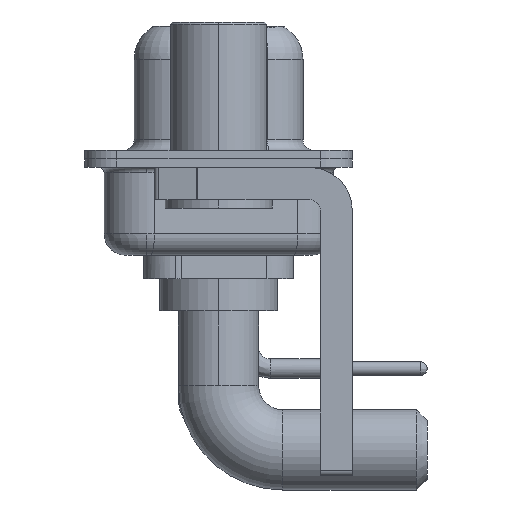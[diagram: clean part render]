
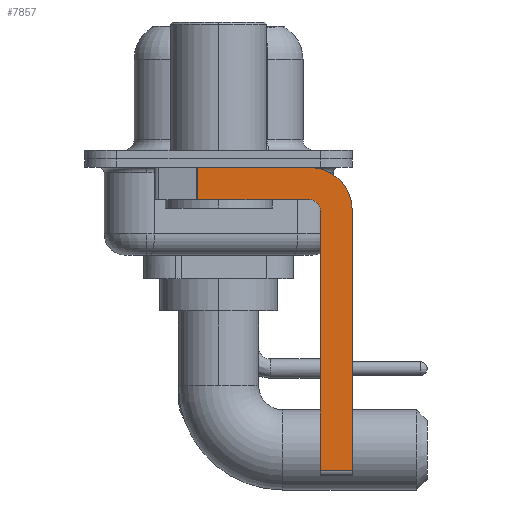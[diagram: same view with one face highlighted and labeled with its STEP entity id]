
A CAD part, left-side view. The second image highlights one B-rep face of the part: STEP entity #7857.
In plain terms, the highlighted planar face has unit normal (-1, 0, 0).
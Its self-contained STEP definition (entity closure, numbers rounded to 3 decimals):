
#25 = CARTESIAN_POINT ( 'NONE',  ( -2.9, -4.25, -0.4 ) ) ;
#339 = CARTESIAN_POINT ( 'NONE',  ( -2.9, -6.25, -2.4 ) ) ;
#407 = VERTEX_POINT ( 'NONE', #7851 ) ;
#475 = VECTOR ( 'NONE', #18164, 1000. ) ;
#522 = CIRCLE ( 'NONE', #15997, 2. ) ;
#2078 = VECTOR ( 'NONE', #6536, 1000. ) ;
#2760 = DIRECTION ( 'NONE',  ( 0., 0., 1. ) ) ;
#2777 = DIRECTION ( 'NONE',  ( 1., 0., 0. ) ) ;
#3137 = ORIENTED_EDGE ( 'NONE', *, *, #11200, .F. ) ;
#3430 = DIRECTION ( 'NONE',  ( 1., 0., 0. ) ) ;
#3454 = DIRECTION ( 'NONE',  ( 0., 0., 1. ) ) ;
#3721 = VERTEX_POINT ( 'NONE', #17785 ) ;
#4011 = EDGE_CURVE ( 'NONE', #407, #14669, #10313, .T. ) ;
#4802 = EDGE_CURVE ( 'NONE', #6082, #14540, #522, .T. ) ;
#5266 = VECTOR ( 'NONE', #23229, 1000. ) ;
#5614 = VECTOR ( 'NONE', #20807, 1000. ) ;
#6082 = VERTEX_POINT ( 'NONE', #25 ) ;
#6085 = DIRECTION ( 'NONE',  ( -1., 0., 0. ) ) ;
#6464 = EDGE_CURVE ( 'NONE', #15797, #6748, #22939, .T. ) ;
#6536 = DIRECTION ( 'NONE',  ( 0., -1., 0. ) ) ;
#6683 = CARTESIAN_POINT ( 'NONE',  ( -2.9, -4.25, -2.4 ) ) ;
#6748 = VERTEX_POINT ( 'NONE', #16519 ) ;
#6986 = DIRECTION ( 'NONE',  ( 0., 1., 0. ) ) ;
#6990 = DIRECTION ( 'NONE',  ( 0., 0., -1. ) ) ;
#7174 = CARTESIAN_POINT ( 'NONE',  ( -2.9, -6.25, -2.4 ) ) ;
#7233 = CARTESIAN_POINT ( 'NONE',  ( -2.9, -4.75, -14.8 ) ) ;
#7406 = EDGE_CURVE ( 'NONE', #15797, #6082, #21449, .T. ) ;
#7851 = CARTESIAN_POINT ( 'NONE',  ( -2.9, -4.75, -2.4 ) ) ;
#7857 = ADVANCED_FACE ( 'NONE', ( #15652 ), #22893, .F. ) ;
#8286 = AXIS2_PLACEMENT_3D ( 'NONE', #6683, #2777, #18986 ) ;
#9037 = ORIENTED_EDGE ( 'NONE', *, *, #7406, .F. ) ;
#10070 = CARTESIAN_POINT ( 'NONE',  ( -2.9, 0.978, -0.4 ) ) ;
#10183 = EDGE_CURVE ( 'NONE', #19823, #407, #23227, .T. ) ;
#10247 = ORIENTED_EDGE ( 'NONE', *, *, #10538, .F. ) ;
#10313 = CIRCLE ( 'NONE', #14113, 0.5 ) ;
#10538 = EDGE_CURVE ( 'NONE', #14669, #6748, #12653, .T. ) ;
#11200 = EDGE_CURVE ( 'NONE', #14540, #3721, #19838, .T. ) ;
#11345 = VECTOR ( 'NONE', #6986, 1000. ) ;
#12142 = CARTESIAN_POINT ( 'NONE',  ( -2.9, 0.978, -1.9 ) ) ;
#12621 = ORIENTED_EDGE ( 'NONE', *, *, #10183, .F. ) ;
#12632 = CARTESIAN_POINT ( 'NONE',  ( -2.9, -4.75, -14.55 ) ) ;
#12653 = LINE ( 'NONE', #17727, #11345 ) ;
#12671 = ORIENTED_EDGE ( 'NONE', *, *, #15857, .T. ) ;
#14113 = AXIS2_PLACEMENT_3D ( 'NONE', #22279, #6085, #2760 ) ;
#14417 = CARTESIAN_POINT ( 'NONE',  ( -2.9, -4.25, -2.4 ) ) ;
#14540 = VERTEX_POINT ( 'NONE', #339 ) ;
#14669 = VERTEX_POINT ( 'NONE', #19959 ) ;
#14674 = CARTESIAN_POINT ( 'NONE',  ( -2.9, 3., -0.4 ) ) ;
#15652 = FACE_OUTER_BOUND ( 'NONE', #16836, .T. ) ;
#15797 = VERTEX_POINT ( 'NONE', #10070 ) ;
#15857 = EDGE_CURVE ( 'NONE', #19823, #3721, #19074, .T. ) ;
#15997 = AXIS2_PLACEMENT_3D ( 'NONE', #14417, #3430, #6990 ) ;
#16519 = CARTESIAN_POINT ( 'NONE',  ( -2.9, 0.978, -1.9 ) ) ;
#16836 = EDGE_LOOP ( 'NONE', ( #9037, #17601, #10247, #20373, #12621, #12671, #3137, #21345 ) ) ;
#17601 = ORIENTED_EDGE ( 'NONE', *, *, #6464, .T. ) ;
#17727 = CARTESIAN_POINT ( 'NONE',  ( -2.9, -4.25, -1.9 ) ) ;
#17785 = CARTESIAN_POINT ( 'NONE',  ( -2.9, -6.25, -14.55 ) ) ;
#18164 = DIRECTION ( 'NONE',  ( 0., 0., -1. ) ) ;
#18986 = DIRECTION ( 'NONE',  ( 0., 0., -1. ) ) ;
#19074 = LINE ( 'NONE', #22744, #2078 ) ;
#19823 = VERTEX_POINT ( 'NONE', #12632 ) ;
#19838 = LINE ( 'NONE', #7174, #475 ) ;
#19959 = CARTESIAN_POINT ( 'NONE',  ( -2.9, -4.25, -1.9 ) ) ;
#20373 = ORIENTED_EDGE ( 'NONE', *, *, #4011, .F. ) ;
#20807 = DIRECTION ( 'NONE',  ( 0., 0., -1. ) ) ;
#21345 = ORIENTED_EDGE ( 'NONE', *, *, #4802, .F. ) ;
#21449 = LINE ( 'NONE', #14674, #5266 ) ;
#22279 = CARTESIAN_POINT ( 'NONE',  ( -2.9, -4.25, -2.4 ) ) ;
#22328 = VECTOR ( 'NONE', #3454, 1000. ) ;
#22744 = CARTESIAN_POINT ( 'NONE',  ( -2.9, -4.25, -14.55 ) ) ;
#22893 = PLANE ( 'NONE',  #8286 ) ;
#22939 = LINE ( 'NONE', #12142, #5614 ) ;
#23227 = LINE ( 'NONE', #7233, #22328 ) ;
#23229 = DIRECTION ( 'NONE',  ( 0., -1., 0. ) ) ;
